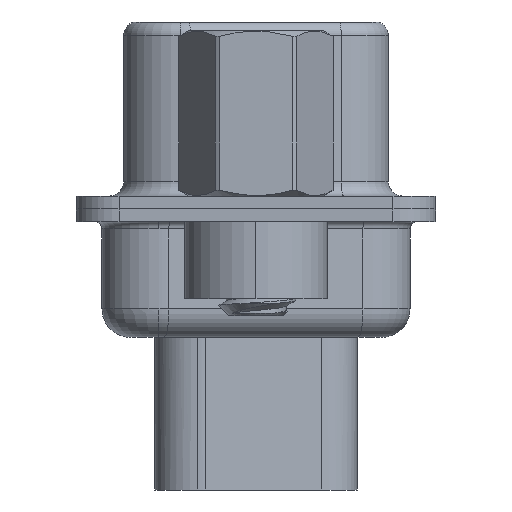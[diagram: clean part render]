
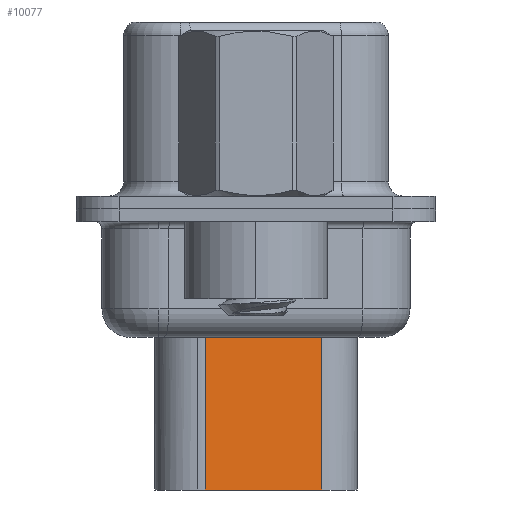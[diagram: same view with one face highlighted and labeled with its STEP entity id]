
A CAD part, left-side view. The second image highlights one B-rep face of the part: STEP entity #10077.
In plain terms, the highlighted planar face has unit normal (-0.985, -0.174, 0).
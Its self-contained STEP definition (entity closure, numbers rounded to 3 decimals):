
#951 = VECTOR ( 'NONE', #9303, 1000. ) ;
#1110 = EDGE_LOOP ( 'NONE', ( #7121, #3321, #17837, #19093 ) ) ;
#2376 = LINE ( 'NONE', #2481, #951 ) ;
#2481 = CARTESIAN_POINT ( 'NONE',  ( 4.338, 2.749, -3.975 ) ) ;
#2926 = CARTESIAN_POINT ( 'NONE',  ( 4.509, 1.78, -3.1 ) ) ;
#3321 = ORIENTED_EDGE ( 'NONE', *, *, #6609, .T. ) ;
#3887 = LINE ( 'NONE', #18988, #17023 ) ;
#6609 = EDGE_CURVE ( 'NONE', #21066, #7344, #2376, .T. ) ;
#7038 = VECTOR ( 'NONE', #13212, 1000. ) ;
#7121 = ORIENTED_EDGE ( 'NONE', *, *, #19874, .F. ) ;
#7344 = VERTEX_POINT ( 'NONE', #20679 ) ;
#8645 = DIRECTION ( 'NONE',  ( -0.174, 0.985, 0. ) ) ;
#8698 = CARTESIAN_POINT ( 'NONE',  ( 4.509, 1.78, -3.1 ) ) ;
#9303 = DIRECTION ( 'NONE',  ( -0.174, 0.985, 0. ) ) ;
#10077 = ADVANCED_FACE ( 'NONE', ( #17104 ), #12053, .T. ) ;
#10379 = DIRECTION ( 'NONE',  ( -0.985, -0.174, 0. ) ) ;
#10803 = DIRECTION ( 'NONE',  ( 0., 0., -1. ) ) ;
#11099 = VERTEX_POINT ( 'NONE', #16336 ) ;
#11722 = CARTESIAN_POINT ( 'NONE',  ( 5.228, -2.3, -3.975 ) ) ;
#12053 = PLANE ( 'NONE',  #19792 ) ;
#13212 = DIRECTION ( 'NONE',  ( 0., 0., -1. ) ) ;
#13799 = CARTESIAN_POINT ( 'NONE',  ( 4.509, 1.78, -9.85 ) ) ;
#14330 = CARTESIAN_POINT ( 'NONE',  ( 5.228, -2.3, -9.85 ) ) ;
#16305 = VECTOR ( 'NONE', #8645, 1000. ) ;
#16336 = CARTESIAN_POINT ( 'NONE',  ( 4.509, 1.78, -9.85 ) ) ;
#16380 = EDGE_CURVE ( 'NONE', #18255, #11099, #17265, .T. ) ;
#16762 = EDGE_CURVE ( 'NONE', #7344, #11099, #18247, .T. ) ;
#17023 = VECTOR ( 'NONE', #10803, 1000. ) ;
#17104 = FACE_OUTER_BOUND ( 'NONE', #1110, .T. ) ;
#17265 = LINE ( 'NONE', #13799, #16305 ) ;
#17837 = ORIENTED_EDGE ( 'NONE', *, *, #16762, .T. ) ;
#18247 = LINE ( 'NONE', #2926, #7038 ) ;
#18255 = VERTEX_POINT ( 'NONE', #14330 ) ;
#18776 = DIRECTION ( 'NONE',  ( 0.174, -0.985, 0. ) ) ;
#18988 = CARTESIAN_POINT ( 'NONE',  ( 5.228, -2.3, -3.1 ) ) ;
#19093 = ORIENTED_EDGE ( 'NONE', *, *, #16380, .F. ) ;
#19792 = AXIS2_PLACEMENT_3D ( 'NONE', #8698, #10379, #18776 ) ;
#19874 = EDGE_CURVE ( 'NONE', #21066, #18255, #3887, .T. ) ;
#20679 = CARTESIAN_POINT ( 'NONE',  ( 4.509, 1.78, -3.975 ) ) ;
#21066 = VERTEX_POINT ( 'NONE', #11722 ) ;
